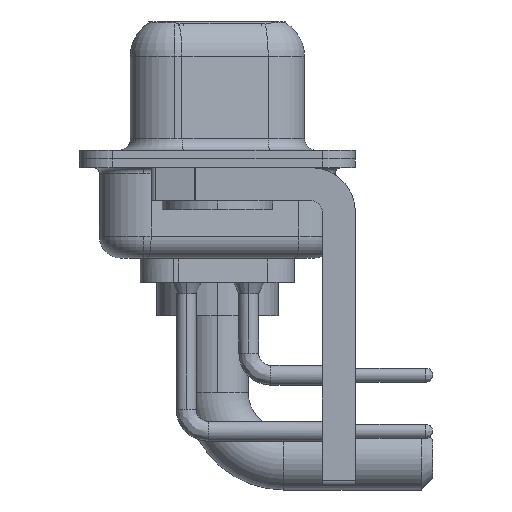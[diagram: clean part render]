
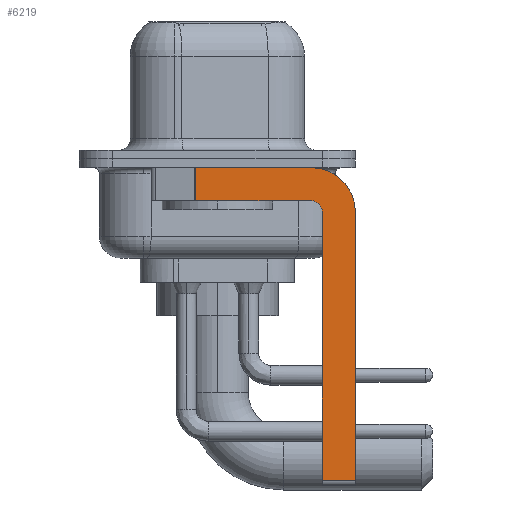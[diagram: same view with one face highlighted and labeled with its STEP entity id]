
A CAD part, left-side view. The second image highlights one B-rep face of the part: STEP entity #6219.
In plain terms, the highlighted planar face has unit normal (-1, 0, 0).
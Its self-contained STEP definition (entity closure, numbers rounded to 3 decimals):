
#485 = VECTOR ( 'NONE', #1967, 1000. ) ;
#554 = VERTEX_POINT ( 'NONE', #7601 ) ;
#885 = ORIENTED_EDGE ( 'NONE', *, *, #5072, .T. ) ;
#1052 = VERTEX_POINT ( 'NONE', #3759 ) ;
#1460 = VERTEX_POINT ( 'NONE', #14132 ) ;
#1617 = ORIENTED_EDGE ( 'NONE', *, *, #12155, .F. ) ;
#1646 = LINE ( 'NONE', #14426, #9152 ) ;
#1848 = VERTEX_POINT ( 'NONE', #10569 ) ;
#1865 = LINE ( 'NONE', #16622, #485 ) ;
#1880 = ORIENTED_EDGE ( 'NONE', *, *, #6932, .T. ) ;
#1967 = DIRECTION ( 'NONE',  ( 0., 0., -1. ) ) ;
#2126 = VERTEX_POINT ( 'NONE', #2482 ) ;
#2168 = EDGE_LOOP ( 'NONE', ( #1617, #1880, #3471, #17481, #18854, #885, #12555, #5843 ) ) ;
#2344 = CARTESIAN_POINT ( 'NONE',  ( -2.9, -4.25, -14.55 ) ) ;
#2482 = CARTESIAN_POINT ( 'NONE',  ( -2.9, 0.978, -1.9 ) ) ;
#2542 = VERTEX_POINT ( 'NONE', #6362 ) ;
#3471 = ORIENTED_EDGE ( 'NONE', *, *, #17208, .F. ) ;
#3759 = CARTESIAN_POINT ( 'NONE',  ( -2.9, -4.25, -1.9 ) ) ;
#3771 = AXIS2_PLACEMENT_3D ( 'NONE', #12135, #7700, #10940 ) ;
#4412 = AXIS2_PLACEMENT_3D ( 'NONE', #8734, #5780, #8636 ) ;
#4983 = VERTEX_POINT ( 'NONE', #11198 ) ;
#5072 = EDGE_CURVE ( 'NONE', #13716, #4983, #11842, .T. ) ;
#5310 = EDGE_CURVE ( 'NONE', #554, #1052, #16010, .T. ) ;
#5485 = DIRECTION ( 'NONE',  ( 0., -1., 0. ) ) ;
#5699 = DIRECTION ( 'NONE',  ( 0., 0., -1. ) ) ;
#5780 = DIRECTION ( 'NONE',  ( 1., 0., 0. ) ) ;
#5843 = ORIENTED_EDGE ( 'NONE', *, *, #18287, .F. ) ;
#6219 = ADVANCED_FACE ( 'NONE', ( #16298 ), #8918, .F. ) ;
#6362 = CARTESIAN_POINT ( 'NONE',  ( -2.9, -4.25, -0.4 ) ) ;
#6467 = CARTESIAN_POINT ( 'NONE',  ( -2.9, 3., -0.4 ) ) ;
#6587 = LINE ( 'NONE', #18295, #17170 ) ;
#6932 = EDGE_CURVE ( 'NONE', #1848, #2126, #1646, .T. ) ;
#7068 = VECTOR ( 'NONE', #16980, 1000. ) ;
#7601 = CARTESIAN_POINT ( 'NONE',  ( -2.9, -4.75, -2.4 ) ) ;
#7700 = DIRECTION ( 'NONE',  ( -1., 0., 0. ) ) ;
#8522 = LINE ( 'NONE', #16202, #16398 ) ;
#8636 = DIRECTION ( 'NONE',  ( 0., 0., -1. ) ) ;
#8734 = CARTESIAN_POINT ( 'NONE',  ( -2.9, -4.25, -2.4 ) ) ;
#8775 = VECTOR ( 'NONE', #5485, 1000. ) ;
#8918 = PLANE ( 'NONE',  #4412 ) ;
#9152 = VECTOR ( 'NONE', #18755, 1000. ) ;
#10320 = CARTESIAN_POINT ( 'NONE',  ( -2.9, -4.25, -2.4 ) ) ;
#10569 = CARTESIAN_POINT ( 'NONE',  ( -2.9, 0.978, -0.4 ) ) ;
#10940 = DIRECTION ( 'NONE',  ( 0., 0., 1. ) ) ;
#11198 = CARTESIAN_POINT ( 'NONE',  ( -2.9, -6.25, -14.55 ) ) ;
#11389 = DIRECTION ( 'NONE',  ( 0., 1., 0. ) ) ;
#11842 = LINE ( 'NONE', #2344, #8775 ) ;
#12135 = CARTESIAN_POINT ( 'NONE',  ( -2.9, -4.25, -2.4 ) ) ;
#12155 = EDGE_CURVE ( 'NONE', #1848, #2542, #18094, .T. ) ;
#12555 = ORIENTED_EDGE ( 'NONE', *, *, #13465, .F. ) ;
#13465 = EDGE_CURVE ( 'NONE', #1460, #4983, #1865, .T. ) ;
#13716 = VERTEX_POINT ( 'NONE', #14043 ) ;
#14043 = CARTESIAN_POINT ( 'NONE',  ( -2.9, -4.75, -14.55 ) ) ;
#14132 = CARTESIAN_POINT ( 'NONE',  ( -2.9, -6.25, -2.4 ) ) ;
#14426 = CARTESIAN_POINT ( 'NONE',  ( -2.9, 0.978, -1.9 ) ) ;
#14751 = EDGE_CURVE ( 'NONE', #13716, #554, #6587, .T. ) ;
#15487 = AXIS2_PLACEMENT_3D ( 'NONE', #10320, #19167, #5699 ) ;
#16010 = CIRCLE ( 'NONE', #3771, 0.5 ) ;
#16202 = CARTESIAN_POINT ( 'NONE',  ( -2.9, -4.25, -1.9 ) ) ;
#16298 = FACE_OUTER_BOUND ( 'NONE', #2168, .T. ) ;
#16398 = VECTOR ( 'NONE', #11389, 1000. ) ;
#16622 = CARTESIAN_POINT ( 'NONE',  ( -2.9, -6.25, -2.4 ) ) ;
#16980 = DIRECTION ( 'NONE',  ( 0., -1., 0. ) ) ;
#17170 = VECTOR ( 'NONE', #18491, 1000. ) ;
#17208 = EDGE_CURVE ( 'NONE', #1052, #2126, #8522, .T. ) ;
#17481 = ORIENTED_EDGE ( 'NONE', *, *, #5310, .F. ) ;
#18094 = LINE ( 'NONE', #6467, #7068 ) ;
#18287 = EDGE_CURVE ( 'NONE', #2542, #1460, #19265, .T. ) ;
#18295 = CARTESIAN_POINT ( 'NONE',  ( -2.9, -4.75, -14.8 ) ) ;
#18491 = DIRECTION ( 'NONE',  ( 0., 0., 1. ) ) ;
#18755 = DIRECTION ( 'NONE',  ( 0., 0., -1. ) ) ;
#18854 = ORIENTED_EDGE ( 'NONE', *, *, #14751, .F. ) ;
#19167 = DIRECTION ( 'NONE',  ( 1., 0., 0. ) ) ;
#19265 = CIRCLE ( 'NONE', #15487, 2. ) ;
